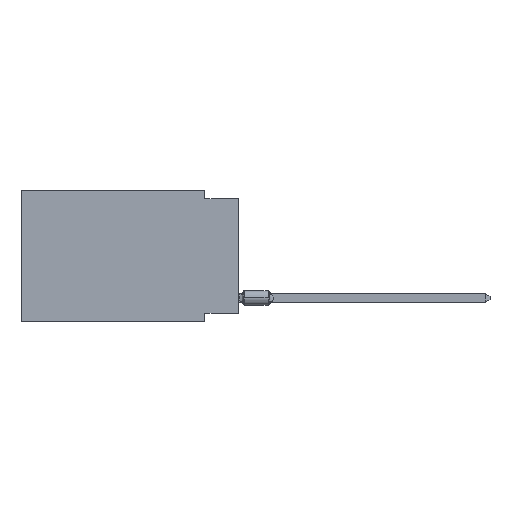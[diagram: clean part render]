
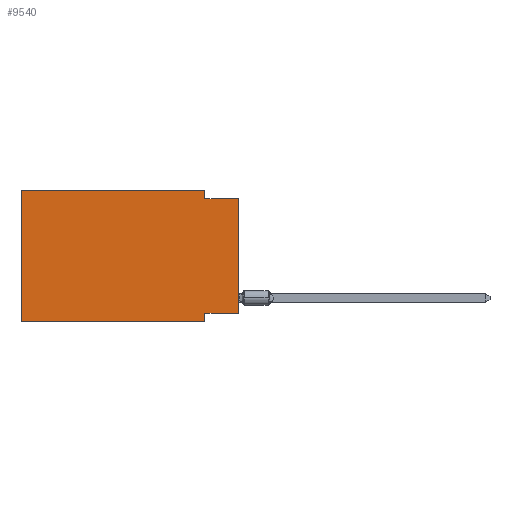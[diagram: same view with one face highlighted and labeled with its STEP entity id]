
A CAD part, left-side view. The second image highlights one B-rep face of the part: STEP entity #9540.
In plain terms, the highlighted planar face has unit normal (-1, 0, 0).
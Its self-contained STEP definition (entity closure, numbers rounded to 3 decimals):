
#321 = DIRECTION ( 'NONE',  ( 0., 0., 1. ) ) ;
#355 = ORIENTED_EDGE ( 'NONE', *, *, #29671, .F. ) ;
#1091 = EDGE_CURVE ( 'NONE', #18678, #30853, #33248, .T. ) ;
#2463 = LINE ( 'NONE', #8360, #21387 ) ;
#2766 = VERTEX_POINT ( 'NONE', #6286 ) ;
#2839 = CARTESIAN_POINT ( 'NONE',  ( 0., 0., -0.635 ) ) ;
#3191 = CARTESIAN_POINT ( 'NONE',  ( 0., 16.383, 0. ) ) ;
#5022 = VECTOR ( 'NONE', #18125, 1000. ) ;
#5349 = VERTEX_POINT ( 'NONE', #6109 ) ;
#6109 = CARTESIAN_POINT ( 'NONE',  ( 0., 2.54, -9.271 ) ) ;
#6286 = CARTESIAN_POINT ( 'NONE',  ( 0., 16.383, -9.906 ) ) ;
#6539 = DIRECTION ( 'NONE',  ( 0., -1., 0. ) ) ;
#6712 = LINE ( 'NONE', #24355, #17642 ) ;
#7679 = ORIENTED_EDGE ( 'NONE', *, *, #33245, .F. ) ;
#8360 = CARTESIAN_POINT ( 'NONE',  ( 0., 16.383, -9.906 ) ) ;
#8743 = CARTESIAN_POINT ( 'NONE',  ( 0., 0., 0. ) ) ;
#8757 = CARTESIAN_POINT ( 'NONE',  ( 0., 0., -9.271 ) ) ;
#9540 = ADVANCED_FACE ( 'NONE', ( #20862 ), #35791, .F. ) ;
#9707 = LINE ( 'NONE', #33656, #5022 ) ;
#10092 = EDGE_CURVE ( 'NONE', #2766, #21918, #6712, .T. ) ;
#11472 = LINE ( 'NONE', #17163, #24352 ) ;
#11965 = VERTEX_POINT ( 'NONE', #21154 ) ;
#13404 = VECTOR ( 'NONE', #38754, 1000. ) ;
#14785 = CARTESIAN_POINT ( 'NONE',  ( 0., 0., -0.635 ) ) ;
#16418 = VECTOR ( 'NONE', #321, 1000. ) ;
#17163 = CARTESIAN_POINT ( 'NONE',  ( 0., 2.54, 0. ) ) ;
#17210 = EDGE_CURVE ( 'NONE', #22962, #30853, #36031, .T. ) ;
#17642 = VECTOR ( 'NONE', #21205, 1000. ) ;
#17846 = CARTESIAN_POINT ( 'NONE',  ( 0., 2.54, 0. ) ) ;
#18125 = DIRECTION ( 'NONE',  ( 0., 1., 0. ) ) ;
#18197 = CARTESIAN_POINT ( 'NONE',  ( 0., 2.54, -0.635 ) ) ;
#18528 = ORIENTED_EDGE ( 'NONE', *, *, #17210, .T. ) ;
#18678 = VERTEX_POINT ( 'NONE', #18197 ) ;
#19243 = ORIENTED_EDGE ( 'NONE', *, *, #1091, .F. ) ;
#19269 = EDGE_LOOP ( 'NONE', ( #18528, #19243, #28768, #7679, #26351, #37020, #355, #30494 ) ) ;
#20862 = FACE_OUTER_BOUND ( 'NONE', #19269, .T. ) ;
#20893 = AXIS2_PLACEMENT_3D ( 'NONE', #33646, #21655, #35994 ) ;
#21154 = CARTESIAN_POINT ( 'NONE',  ( 0., 2.54, -9.906 ) ) ;
#21205 = DIRECTION ( 'NONE',  ( 0., 0., 1. ) ) ;
#21387 = VECTOR ( 'NONE', #26406, 1000. ) ;
#21655 = DIRECTION ( 'NONE',  ( 1., 0., 0. ) ) ;
#21701 = EDGE_CURVE ( 'NONE', #22962, #5349, #9707, .T. ) ;
#21918 = VERTEX_POINT ( 'NONE', #38324 ) ;
#22962 = VERTEX_POINT ( 'NONE', #8757 ) ;
#23397 = EDGE_CURVE ( 'NONE', #36958, #18678, #11472, .T. ) ;
#24352 = VECTOR ( 'NONE', #32472, 1000. ) ;
#24355 = CARTESIAN_POINT ( 'NONE',  ( 0., 16.383, 0. ) ) ;
#25175 = LINE ( 'NONE', #31076, #25938 ) ;
#25938 = VECTOR ( 'NONE', #31657, 1000. ) ;
#26230 = EDGE_CURVE ( 'NONE', #2766, #11965, #2463, .T. ) ;
#26351 = ORIENTED_EDGE ( 'NONE', *, *, #10092, .F. ) ;
#26406 = DIRECTION ( 'NONE',  ( 0., -1., 0. ) ) ;
#28768 = ORIENTED_EDGE ( 'NONE', *, *, #23397, .F. ) ;
#29671 = EDGE_CURVE ( 'NONE', #5349, #11965, #25175, .T. ) ;
#30494 = ORIENTED_EDGE ( 'NONE', *, *, #21701, .F. ) ;
#30853 = VERTEX_POINT ( 'NONE', #2839 ) ;
#31076 = CARTESIAN_POINT ( 'NONE',  ( 0., 2.54, -9.906 ) ) ;
#31657 = DIRECTION ( 'NONE',  ( 0., 0., -1. ) ) ;
#32472 = DIRECTION ( 'NONE',  ( 0., 0., -1. ) ) ;
#33245 = EDGE_CURVE ( 'NONE', #21918, #36958, #33430, .T. ) ;
#33248 = LINE ( 'NONE', #14785, #13404 ) ;
#33430 = LINE ( 'NONE', #3191, #35283 ) ;
#33646 = CARTESIAN_POINT ( 'NONE',  ( 0., 16.383, 0. ) ) ;
#33656 = CARTESIAN_POINT ( 'NONE',  ( 0., 0., -9.271 ) ) ;
#35283 = VECTOR ( 'NONE', #6539, 1000. ) ;
#35791 = PLANE ( 'NONE',  #20893 ) ;
#35994 = DIRECTION ( 'NONE',  ( 0., 0., -1. ) ) ;
#36031 = LINE ( 'NONE', #8743, #16418 ) ;
#36958 = VERTEX_POINT ( 'NONE', #17846 ) ;
#37020 = ORIENTED_EDGE ( 'NONE', *, *, #26230, .T. ) ;
#38324 = CARTESIAN_POINT ( 'NONE',  ( 0., 16.383, 0. ) ) ;
#38754 = DIRECTION ( 'NONE',  ( 0., -1., 0. ) ) ;
